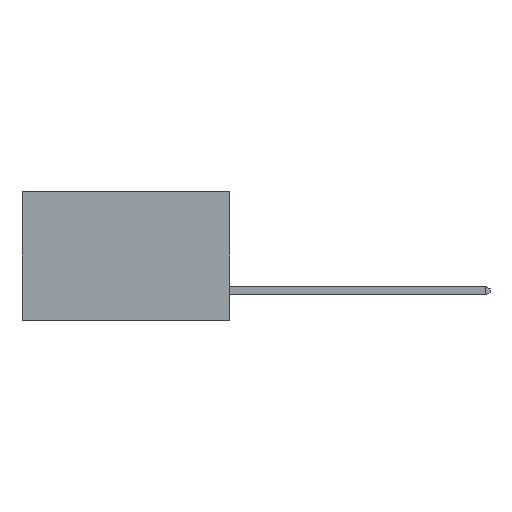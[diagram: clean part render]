
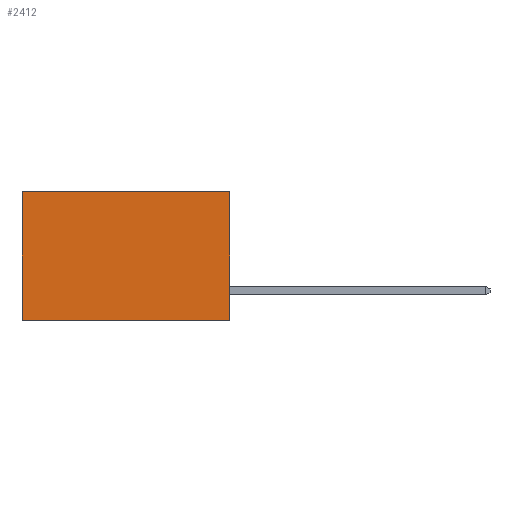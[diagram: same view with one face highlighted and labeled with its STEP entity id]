
A CAD part, left-side view. The second image highlights one B-rep face of the part: STEP entity #2412.
In plain terms, the highlighted planar face has unit normal (-1, 0, 0).
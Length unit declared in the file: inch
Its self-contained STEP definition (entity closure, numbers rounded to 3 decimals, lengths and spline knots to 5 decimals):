
#29 = VERTEX_POINT ( 'NONE', #5052 ) ;
#596 = EDGE_CURVE ( 'NONE', #3164, #29, #2194, .T. ) ;
#885 = VECTOR ( 'NONE', #9506, 39.37008 ) ;
#1586 = DIRECTION ( 'NONE',  ( 0., 0., -1. ) ) ;
#1982 = VECTOR ( 'NONE', #7581, 39.37008 ) ;
#2194 = LINE ( 'NONE', #9091, #8097 ) ;
#2365 = EDGE_CURVE ( 'NONE', #29, #3392, #3045, .T. ) ;
#2412 = ADVANCED_FACE ( 'NONE', ( #6664 ), #6739, .F. ) ;
#3045 = LINE ( 'NONE', #5620, #885 ) ;
#3164 = VERTEX_POINT ( 'NONE', #10025 ) ;
#3392 = VERTEX_POINT ( 'NONE', #5857 ) ;
#3698 = LINE ( 'NONE', #4783, #3935 ) ;
#3935 = VECTOR ( 'NONE', #1586, 39.37008 ) ;
#4584 = VERTEX_POINT ( 'NONE', #6759 ) ;
#4710 = ORIENTED_EDGE ( 'NONE', *, *, #7371, .T. ) ;
#4783 = CARTESIAN_POINT ( 'NONE',  ( 0.298, 0.6, 0. ) ) ;
#5052 = CARTESIAN_POINT ( 'NONE',  ( 0.298, 0., -0.37 ) ) ;
#5164 = EDGE_CURVE ( 'NONE', #3164, #4584, #8374, .T. ) ;
#5620 = CARTESIAN_POINT ( 'NONE',  ( 0.298, 0., -0.37 ) ) ;
#5727 = DIRECTION ( 'NONE',  ( 0., 0., -1. ) ) ;
#5857 = CARTESIAN_POINT ( 'NONE',  ( 0.298, 0.6, -0.37 ) ) ;
#6202 = ORIENTED_EDGE ( 'NONE', *, *, #2365, .F. ) ;
#6316 = AXIS2_PLACEMENT_3D ( 'NONE', #7074, #7929, #5727 ) ;
#6664 = FACE_OUTER_BOUND ( 'NONE', #8098, .T. ) ;
#6739 = PLANE ( 'NONE',  #6316 ) ;
#6759 = CARTESIAN_POINT ( 'NONE',  ( 0.298, 0.6, 0. ) ) ;
#6931 = ORIENTED_EDGE ( 'NONE', *, *, #5164, .T. ) ;
#7074 = CARTESIAN_POINT ( 'NONE',  ( 0.298, 0., 0. ) ) ;
#7371 = EDGE_CURVE ( 'NONE', #4584, #3392, #3698, .T. ) ;
#7518 = ORIENTED_EDGE ( 'NONE', *, *, #596, .F. ) ;
#7581 = DIRECTION ( 'NONE',  ( 0., 1., 0. ) ) ;
#7929 = DIRECTION ( 'NONE',  ( 1., 0., 0. ) ) ;
#8097 = VECTOR ( 'NONE', #8904, 39.37008 ) ;
#8098 = EDGE_LOOP ( 'NONE', ( #4710, #6202, #7518, #6931 ) ) ;
#8374 = LINE ( 'NONE', #9691, #1982 ) ;
#8904 = DIRECTION ( 'NONE',  ( 0., 0., -1. ) ) ;
#9091 = CARTESIAN_POINT ( 'NONE',  ( 0.298, 0., 0. ) ) ;
#9506 = DIRECTION ( 'NONE',  ( 0., 1., 0. ) ) ;
#9691 = CARTESIAN_POINT ( 'NONE',  ( 0.298, 0., 0. ) ) ;
#10025 = CARTESIAN_POINT ( 'NONE',  ( 0.298, 0., 0. ) ) ;
